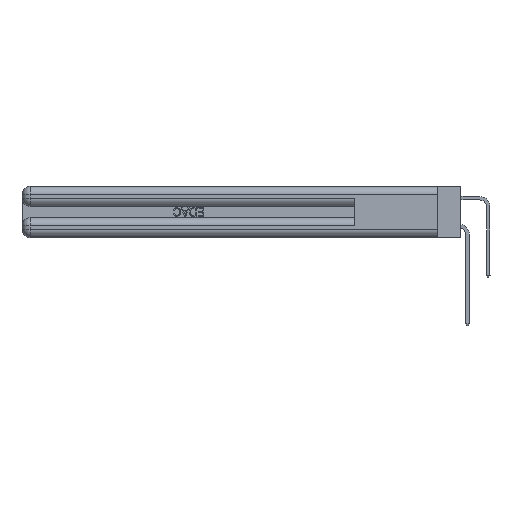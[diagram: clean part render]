
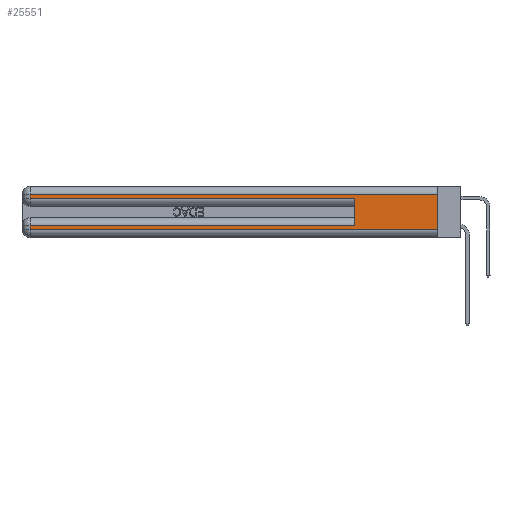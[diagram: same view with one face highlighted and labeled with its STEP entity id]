
A CAD part, left-side view. The second image highlights one B-rep face of the part: STEP entity #25551.
In plain terms, the highlighted planar face has unit normal (-1, 0, 0).
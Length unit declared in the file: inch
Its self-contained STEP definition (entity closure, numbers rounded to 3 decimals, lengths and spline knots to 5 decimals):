
#1992 = LINE ( 'NONE', #19045, #20487 ) ;
#2033 = CARTESIAN_POINT ( 'NONE',  ( 0., 0., 0.06 ) ) ;
#2210 = ORIENTED_EDGE ( 'NONE', *, *, #41708, .T. ) ;
#2879 = DIRECTION ( 'NONE',  ( 0., -1., 0. ) ) ;
#3167 = CARTESIAN_POINT ( 'NONE',  ( 0., 0., 0.37 ) ) ;
#3403 = CARTESIAN_POINT ( 'NONE',  ( 0., 0., 0.37 ) ) ;
#3550 = VERTEX_POINT ( 'NONE', #37943 ) ;
#3932 = LINE ( 'NONE', #5390, #22430 ) ;
#4926 = DIRECTION ( 'NONE',  ( 0., 1., 0. ) ) ;
#5390 = CARTESIAN_POINT ( 'NONE',  ( 0., 2.94, 0.37 ) ) ;
#5473 = EDGE_CURVE ( 'NONE', #39191, #3550, #20248, .T. ) ;
#6278 = VECTOR ( 'NONE', #43443, 39.37008 ) ;
#6898 = PLANE ( 'NONE',  #39744 ) ;
#7529 = LINE ( 'NONE', #21131, #34981 ) ;
#7605 = FACE_OUTER_BOUND ( 'NONE', #41360, .T. ) ;
#9611 = CARTESIAN_POINT ( 'NONE',  ( 0., 0., 0.285 ) ) ;
#10890 = ORIENTED_EDGE ( 'NONE', *, *, #32905, .T. ) ;
#11003 = VECTOR ( 'NONE', #20978, 39.37008 ) ;
#12591 = CARTESIAN_POINT ( 'NONE',  ( 0., 0.6, 0.145 ) ) ;
#12734 = VERTEX_POINT ( 'NONE', #24441 ) ;
#13320 = DIRECTION ( 'NONE',  ( 0., 0., -1. ) ) ;
#13860 = DIRECTION ( 'NONE',  ( 0., 0., -1. ) ) ;
#15446 = VECTOR ( 'NONE', #13320, 39.37008 ) ;
#15510 = LINE ( 'NONE', #12591, #6278 ) ;
#16200 = EDGE_CURVE ( 'NONE', #24404, #12734, #7529, .T. ) ;
#17422 = CARTESIAN_POINT ( 'NONE',  ( 0., 0.6, 0.085 ) ) ;
#17425 = ORIENTED_EDGE ( 'NONE', *, *, #40296, .F. ) ;
#17938 = ORIENTED_EDGE ( 'NONE', *, *, #16200, .T. ) ;
#18651 = VECTOR ( 'NONE', #4926, 39.37008 ) ;
#19045 = CARTESIAN_POINT ( 'NONE',  ( 0., 0., 0.06 ) ) ;
#20248 = LINE ( 'NONE', #37949, #11003 ) ;
#20487 = VECTOR ( 'NONE', #42916, 39.37008 ) ;
#20978 = DIRECTION ( 'NONE',  ( 0., 0., -1. ) ) ;
#21131 = CARTESIAN_POINT ( 'NONE',  ( 0., 0., 0.31 ) ) ;
#22308 = ORIENTED_EDGE ( 'NONE', *, *, #36580, .T. ) ;
#22430 = VECTOR ( 'NONE', #29591, 39.37008 ) ;
#24404 = VERTEX_POINT ( 'NONE', #42089 ) ;
#24441 = CARTESIAN_POINT ( 'NONE',  ( 0., 2.94, 0.31 ) ) ;
#24686 = LINE ( 'NONE', #3167, #15446 ) ;
#25551 = ADVANCED_FACE ( 'NONE', ( #7605 ), #6898, .F. ) ;
#26623 = VECTOR ( 'NONE', #2879, 39.37008 ) ;
#27034 = CARTESIAN_POINT ( 'NONE',  ( 0., 0.6, 0.285 ) ) ;
#27537 = CARTESIAN_POINT ( 'NONE',  ( 0., 2.94, 0.085 ) ) ;
#27852 = LINE ( 'NONE', #29161, #18651 ) ;
#29161 = CARTESIAN_POINT ( 'NONE',  ( 0., 0., 0.085 ) ) ;
#29591 = DIRECTION ( 'NONE',  ( 0., 0., -1. ) ) ;
#31315 = VERTEX_POINT ( 'NONE', #27034 ) ;
#31937 = ORIENTED_EDGE ( 'NONE', *, *, #5473, .T. ) ;
#31986 = EDGE_CURVE ( 'NONE', #24404, #35918, #24686, .T. ) ;
#32905 = EDGE_CURVE ( 'NONE', #12734, #34397, #3932, .T. ) ;
#32972 = ORIENTED_EDGE ( 'NONE', *, *, #31986, .F. ) ;
#34397 = VERTEX_POINT ( 'NONE', #37153 ) ;
#34454 = DIRECTION ( 'NONE',  ( 1., 0., 0. ) ) ;
#34567 = LINE ( 'NONE', #9611, #26623 ) ;
#34981 = VECTOR ( 'NONE', #41503, 39.37008 ) ;
#35918 = VERTEX_POINT ( 'NONE', #2033 ) ;
#36580 = EDGE_CURVE ( 'NONE', #34397, #31315, #34567, .T. ) ;
#37153 = CARTESIAN_POINT ( 'NONE',  ( 0., 2.94, 0.285 ) ) ;
#37330 = VERTEX_POINT ( 'NONE', #17422 ) ;
#37943 = CARTESIAN_POINT ( 'NONE',  ( 0., 2.94, 0.06 ) ) ;
#37949 = CARTESIAN_POINT ( 'NONE',  ( 0., 2.94, 0.37 ) ) ;
#39191 = VERTEX_POINT ( 'NONE', #27537 ) ;
#39513 = EDGE_CURVE ( 'NONE', #3550, #35918, #1992, .T. ) ;
#39744 = AXIS2_PLACEMENT_3D ( 'NONE', #3403, #34454, #13860 ) ;
#40296 = EDGE_CURVE ( 'NONE', #37330, #31315, #15510, .T. ) ;
#41360 = EDGE_LOOP ( 'NONE', ( #32972, #17938, #10890, #22308, #17425, #2210, #31937, #43095 ) ) ;
#41503 = DIRECTION ( 'NONE',  ( 0., 1., 0. ) ) ;
#41708 = EDGE_CURVE ( 'NONE', #37330, #39191, #27852, .T. ) ;
#42089 = CARTESIAN_POINT ( 'NONE',  ( 0., 0., 0.31 ) ) ;
#42916 = DIRECTION ( 'NONE',  ( 0., -1., 0. ) ) ;
#43095 = ORIENTED_EDGE ( 'NONE', *, *, #39513, .T. ) ;
#43443 = DIRECTION ( 'NONE',  ( 0., 0., 1. ) ) ;
